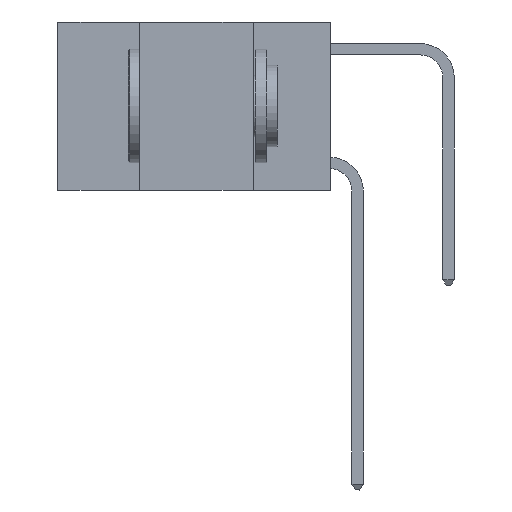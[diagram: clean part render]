
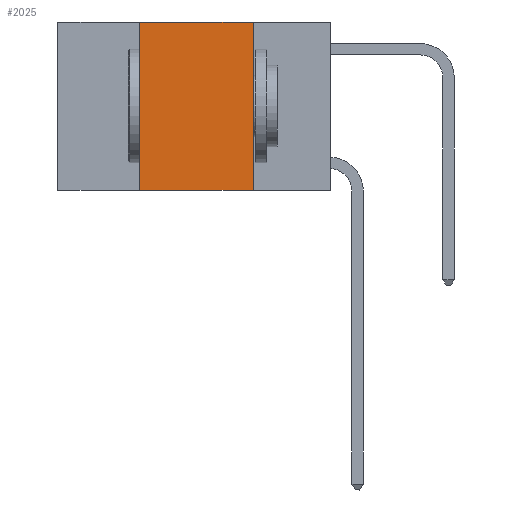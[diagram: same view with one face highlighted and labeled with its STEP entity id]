
A CAD part, left-side view. The second image highlights one B-rep face of the part: STEP entity #2025.
In plain terms, the highlighted planar face has unit normal (-1, 0, 0).
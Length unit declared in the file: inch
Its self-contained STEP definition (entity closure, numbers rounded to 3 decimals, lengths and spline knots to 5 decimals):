
#60 = LINE ( 'NONE', #6379, #9160 ) ;
#172 = CARTESIAN_POINT ( 'NONE',  ( 0., 0.17, -0.37 ) ) ;
#517 = CARTESIAN_POINT ( 'NONE',  ( 0., 0.6, 0. ) ) ;
#521 = CARTESIAN_POINT ( 'NONE',  ( 0., 0.17, 0. ) ) ;
#1161 = VERTEX_POINT ( 'NONE', #521 ) ;
#1235 = CARTESIAN_POINT ( 'NONE',  ( 0., 0.6, 0. ) ) ;
#1395 = DIRECTION ( 'NONE',  ( 0., -1., 0. ) ) ;
#1515 = VECTOR ( 'NONE', #10582, 39.37008 ) ;
#1676 = AXIS2_PLACEMENT_3D ( 'NONE', #517, #6129, #2257 ) ;
#1732 = ORIENTED_EDGE ( 'NONE', *, *, #8475, .T. ) ;
#1897 = FACE_OUTER_BOUND ( 'NONE', #5801, .T. ) ;
#2025 = ADVANCED_FACE ( 'NONE', ( #1897 ), #7400, .F. ) ;
#2120 = DIRECTION ( 'NONE',  ( 0., -1., 0. ) ) ;
#2257 = DIRECTION ( 'NONE',  ( 0., 0., -1. ) ) ;
#2528 = ORIENTED_EDGE ( 'NONE', *, *, #8984, .F. ) ;
#4314 = LINE ( 'NONE', #9868, #1515 ) ;
#4738 = ORIENTED_EDGE ( 'NONE', *, *, #9389, .F. ) ;
#5001 = LINE ( 'NONE', #1235, #5269 ) ;
#5269 = VECTOR ( 'NONE', #1395, 39.37008 ) ;
#5779 = CARTESIAN_POINT ( 'NONE',  ( 0., 0.42, -0.37 ) ) ;
#5801 = EDGE_LOOP ( 'NONE', ( #2528, #10801, #4738, #1732 ) ) ;
#6129 = DIRECTION ( 'NONE',  ( 1., 0., 0. ) ) ;
#6379 = CARTESIAN_POINT ( 'NONE',  ( 0., 0.6, -0.37 ) ) ;
#7400 = PLANE ( 'NONE',  #1676 ) ;
#8108 = CARTESIAN_POINT ( 'NONE',  ( 0., 0.42, 0. ) ) ;
#8363 = DIRECTION ( 'NONE',  ( 0., 0., -1. ) ) ;
#8475 = EDGE_CURVE ( 'NONE', #9706, #9089, #60, .T. ) ;
#8694 = LINE ( 'NONE', #9223, #10283 ) ;
#8984 = EDGE_CURVE ( 'NONE', #1161, #9089, #8694, .T. ) ;
#9089 = VERTEX_POINT ( 'NONE', #172 ) ;
#9160 = VECTOR ( 'NONE', #2120, 39.37008 ) ;
#9223 = CARTESIAN_POINT ( 'NONE',  ( 0., 0.17, 0. ) ) ;
#9389 = EDGE_CURVE ( 'NONE', #9706, #9646, #4314, .T. ) ;
#9564 = EDGE_CURVE ( 'NONE', #9646, #1161, #5001, .T. ) ;
#9646 = VERTEX_POINT ( 'NONE', #8108 ) ;
#9706 = VERTEX_POINT ( 'NONE', #5779 ) ;
#9868 = CARTESIAN_POINT ( 'NONE',  ( 0., 0.42, 0. ) ) ;
#10283 = VECTOR ( 'NONE', #8363, 39.37008 ) ;
#10582 = DIRECTION ( 'NONE',  ( 0., 0., 1. ) ) ;
#10801 = ORIENTED_EDGE ( 'NONE', *, *, #9564, .F. ) ;
